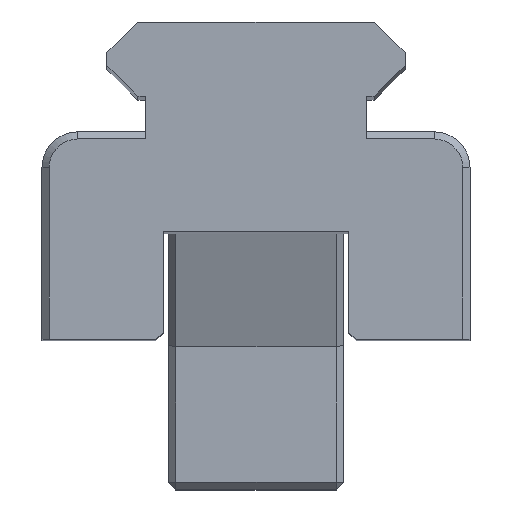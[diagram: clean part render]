
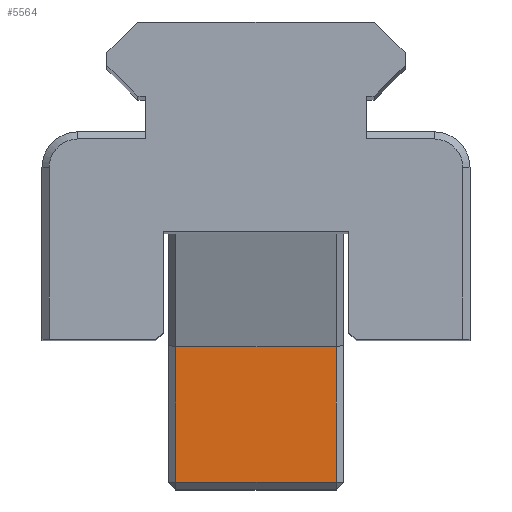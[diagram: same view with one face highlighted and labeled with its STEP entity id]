
A CAD part, top view. The second image highlights one B-rep face of the part: STEP entity #5564.
In plain terms, the highlighted planar face has unit normal (0, 0, 1).
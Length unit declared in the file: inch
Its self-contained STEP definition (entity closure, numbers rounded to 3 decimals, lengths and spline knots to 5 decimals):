
#621 = VECTOR ( 'NONE', #2109, 39.37008 ) ;
#634 = VECTOR ( 'NONE', #4509, 39.37008 ) ;
#899 = LINE ( 'NONE', #1802, #1420 ) ;
#957 = DIRECTION ( 'NONE',  ( 0., -1., 0. ) ) ;
#1420 = VECTOR ( 'NONE', #6359, 39.37008 ) ;
#1552 = DIRECTION ( 'NONE',  ( 0., 0., -1. ) ) ;
#1577 = VERTEX_POINT ( 'NONE', #4768 ) ;
#1618 = CARTESIAN_POINT ( 'NONE',  ( 0.225, 1.07, -6.34 ) ) ;
#1635 = CARTESIAN_POINT ( 'NONE',  ( -0.225, 1.45, -6.34 ) ) ;
#1802 = CARTESIAN_POINT ( 'NONE',  ( 0.225, 1.45, -6.34 ) ) ;
#2008 = VERTEX_POINT ( 'NONE', #1618 ) ;
#2109 = DIRECTION ( 'NONE',  ( 1., 0., 0. ) ) ;
#2481 = VECTOR ( 'NONE', #957, 39.37008 ) ;
#2669 = EDGE_CURVE ( 'NONE', #2008, #4721, #899, .T. ) ;
#2928 = ORIENTED_EDGE ( 'NONE', *, *, #6259, .T. ) ;
#3170 = VERTEX_POINT ( 'NONE', #1635 ) ;
#3307 = AXIS2_PLACEMENT_3D ( 'NONE', #5548, #1552, #3932 ) ;
#3808 = CARTESIAN_POINT ( 'NONE',  ( -0.225, 1.05, -6.34 ) ) ;
#3932 = DIRECTION ( 'NONE',  ( -1., 0., 0. ) ) ;
#3995 = FACE_OUTER_BOUND ( 'NONE', #4418, .T. ) ;
#4144 = CARTESIAN_POINT ( 'NONE',  ( 0.245, 1.07, -6.34 ) ) ;
#4368 = CARTESIAN_POINT ( 'NONE',  ( 0.225, 1.45, -6.34 ) ) ;
#4409 = EDGE_CURVE ( 'NONE', #1577, #2008, #4606, .T. ) ;
#4418 = EDGE_LOOP ( 'NONE', ( #5943, #6104, #5200, #2928 ) ) ;
#4509 = DIRECTION ( 'NONE',  ( 1., 0., 0. ) ) ;
#4606 = LINE ( 'NONE', #4144, #634 ) ;
#4721 = VERTEX_POINT ( 'NONE', #4368 ) ;
#4768 = CARTESIAN_POINT ( 'NONE',  ( -0.225, 1.07, -6.34 ) ) ;
#4982 = CARTESIAN_POINT ( 'NONE',  ( -0.59877, 1.45, -6.34 ) ) ;
#5074 = LINE ( 'NONE', #4982, #621 ) ;
#5200 = ORIENTED_EDGE ( 'NONE', *, *, #5233, .F. ) ;
#5233 = EDGE_CURVE ( 'NONE', #3170, #4721, #5074, .T. ) ;
#5408 = LINE ( 'NONE', #3808, #2481 ) ;
#5548 = CARTESIAN_POINT ( 'NONE',  ( -0.59877, 1.05, -6.34 ) ) ;
#5564 = ADVANCED_FACE ( 'NONE', ( #3995 ), #5947, .F. ) ;
#5943 = ORIENTED_EDGE ( 'NONE', *, *, #4409, .T. ) ;
#5947 = PLANE ( 'NONE',  #3307 ) ;
#6104 = ORIENTED_EDGE ( 'NONE', *, *, #2669, .T. ) ;
#6259 = EDGE_CURVE ( 'NONE', #3170, #1577, #5408, .T. ) ;
#6359 = DIRECTION ( 'NONE',  ( 0., 1., 0. ) ) ;
